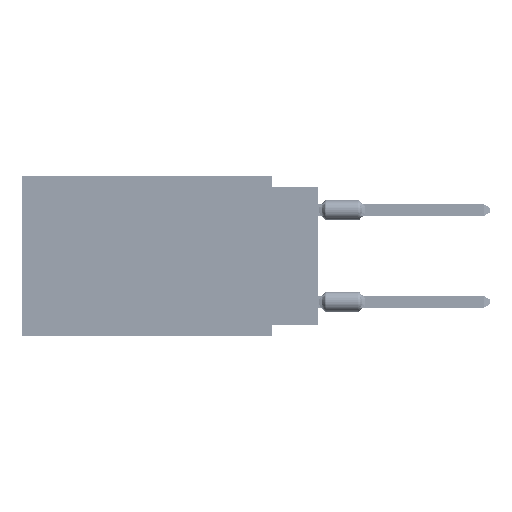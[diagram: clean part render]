
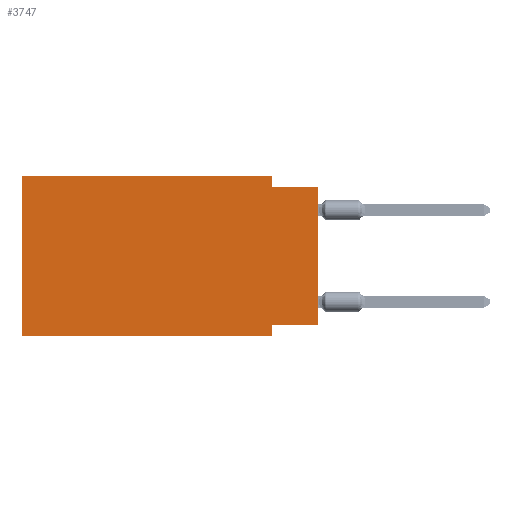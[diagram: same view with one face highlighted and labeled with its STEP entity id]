
A CAD part, left-side view. The second image highlights one B-rep face of the part: STEP entity #3747.
In plain terms, the highlighted planar face has unit normal (-1, 0, 0).
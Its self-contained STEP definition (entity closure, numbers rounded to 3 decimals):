
#1066 = CARTESIAN_POINT ( 'NONE',  ( 0., 0., -8.255 ) ) ;
#1695 = EDGE_CURVE ( 'NONE', #24965, #8599, #10857, .T. ) ;
#2765 = EDGE_CURVE ( 'NONE', #7435, #68412, #64762, .T. ) ;
#3187 = CARTESIAN_POINT ( 'NONE',  ( 0., 16.383, 0. ) ) ;
#3747 = ADVANCED_FACE ( 'NONE', ( #74091 ), #66542, .F. ) ;
#6079 = CARTESIAN_POINT ( 'NONE',  ( 0., 2.54, -8.255 ) ) ;
#6703 = CARTESIAN_POINT ( 'NONE',  ( 0., 16.383, 0. ) ) ;
#7435 = VERTEX_POINT ( 'NONE', #54149 ) ;
#7863 = ORIENTED_EDGE ( 'NONE', *, *, #78974, .F. ) ;
#8599 = VERTEX_POINT ( 'NONE', #20557 ) ;
#10857 = LINE ( 'NONE', #75130, #63582 ) ;
#11036 = EDGE_CURVE ( 'NONE', #7435, #17051, #19717, .T. ) ;
#11330 = ORIENTED_EDGE ( 'NONE', *, *, #76396, .F. ) ;
#11666 = AXIS2_PLACEMENT_3D ( 'NONE', #79978, #47646, #28714 ) ;
#12576 = DIRECTION ( 'NONE',  ( 0., 0., 1. ) ) ;
#13069 = CARTESIAN_POINT ( 'NONE',  ( 0., 16.383, -8.89 ) ) ;
#14148 = DIRECTION ( 'NONE',  ( 0., 1., 0. ) ) ;
#14237 = VECTOR ( 'NONE', #82426, 1000. ) ;
#15278 = VERTEX_POINT ( 'NONE', #47720 ) ;
#17051 = VERTEX_POINT ( 'NONE', #3187 ) ;
#18088 = ORIENTED_EDGE ( 'NONE', *, *, #2765, .T. ) ;
#19717 = LINE ( 'NONE', #6703, #70333 ) ;
#20557 = CARTESIAN_POINT ( 'NONE',  ( 0., 0., -0.635 ) ) ;
#21093 = EDGE_CURVE ( 'NONE', #55402, #8599, #68437, .T. ) ;
#22066 = ORIENTED_EDGE ( 'NONE', *, *, #11036, .F. ) ;
#23482 = DIRECTION ( 'NONE',  ( 0., 0., 1. ) ) ;
#23853 = LINE ( 'NONE', #75523, #78486 ) ;
#23931 = EDGE_CURVE ( 'NONE', #15278, #24965, #39849, .T. ) ;
#24265 = DIRECTION ( 'NONE',  ( 0., 0., -1. ) ) ;
#24965 = VERTEX_POINT ( 'NONE', #59836 ) ;
#25460 = EDGE_LOOP ( 'NONE', ( #57358, #75774, #49839, #7863, #22066, #18088, #11330, #53451 ) ) ;
#28714 = DIRECTION ( 'NONE',  ( 0., 0., -1. ) ) ;
#37633 = CARTESIAN_POINT ( 'NONE',  ( 0., 2.54, -8.89 ) ) ;
#39849 = LINE ( 'NONE', #40274, #73708 ) ;
#40274 = CARTESIAN_POINT ( 'NONE',  ( 0., 2.54, 0. ) ) ;
#45569 = DIRECTION ( 'NONE',  ( 0., -1., 0. ) ) ;
#46105 = EDGE_CURVE ( 'NONE', #55402, #76898, #71306, .T. ) ;
#46588 = DIRECTION ( 'NONE',  ( 0., 0., -1. ) ) ;
#47646 = DIRECTION ( 'NONE',  ( 1., 0., 0. ) ) ;
#47720 = CARTESIAN_POINT ( 'NONE',  ( 0., 2.54, 0. ) ) ;
#49839 = ORIENTED_EDGE ( 'NONE', *, *, #23931, .F. ) ;
#53451 = ORIENTED_EDGE ( 'NONE', *, *, #46105, .F. ) ;
#54149 = CARTESIAN_POINT ( 'NONE',  ( 0., 16.383, -8.89 ) ) ;
#54589 = DIRECTION ( 'NONE',  ( 0., -1., 0. ) ) ;
#55402 = VERTEX_POINT ( 'NONE', #1066 ) ;
#57358 = ORIENTED_EDGE ( 'NONE', *, *, #21093, .T. ) ;
#59140 = CARTESIAN_POINT ( 'NONE',  ( 0., 0., -8.255 ) ) ;
#59836 = CARTESIAN_POINT ( 'NONE',  ( 0., 2.54, -0.635 ) ) ;
#63238 = LINE ( 'NONE', #77505, #76081 ) ;
#63370 = CARTESIAN_POINT ( 'NONE',  ( 0., 0., 0. ) ) ;
#63582 = VECTOR ( 'NONE', #54589, 1000. ) ;
#64762 = LINE ( 'NONE', #13069, #14237 ) ;
#66542 = PLANE ( 'NONE',  #11666 ) ;
#68412 = VERTEX_POINT ( 'NONE', #37633 ) ;
#68437 = LINE ( 'NONE', #63370, #68619 ) ;
#68619 = VECTOR ( 'NONE', #23482, 1000. ) ;
#70333 = VECTOR ( 'NONE', #12576, 1000. ) ;
#71306 = LINE ( 'NONE', #59140, #81299 ) ;
#73708 = VECTOR ( 'NONE', #46588, 1000. ) ;
#74091 = FACE_OUTER_BOUND ( 'NONE', #25460, .T. ) ;
#75130 = CARTESIAN_POINT ( 'NONE',  ( 0., 0., -0.635 ) ) ;
#75523 = CARTESIAN_POINT ( 'NONE',  ( 0., 2.54, -8.89 ) ) ;
#75774 = ORIENTED_EDGE ( 'NONE', *, *, #1695, .F. ) ;
#76081 = VECTOR ( 'NONE', #45569, 1000. ) ;
#76396 = EDGE_CURVE ( 'NONE', #76898, #68412, #23853, .T. ) ;
#76898 = VERTEX_POINT ( 'NONE', #6079 ) ;
#77505 = CARTESIAN_POINT ( 'NONE',  ( 0., 16.383, 0. ) ) ;
#78486 = VECTOR ( 'NONE', #24265, 1000. ) ;
#78974 = EDGE_CURVE ( 'NONE', #17051, #15278, #63238, .T. ) ;
#79978 = CARTESIAN_POINT ( 'NONE',  ( 0., 16.383, 0. ) ) ;
#81299 = VECTOR ( 'NONE', #14148, 1000. ) ;
#82426 = DIRECTION ( 'NONE',  ( 0., -1., 0. ) ) ;
